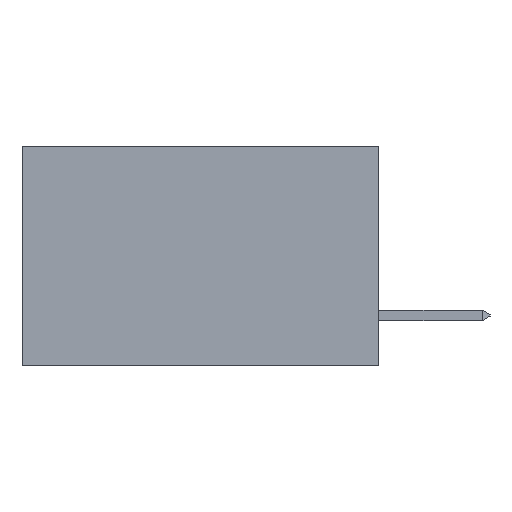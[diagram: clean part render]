
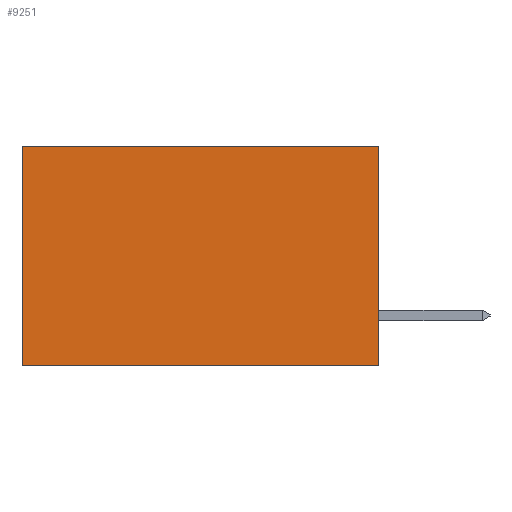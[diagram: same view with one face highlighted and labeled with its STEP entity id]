
A CAD part, left-side view. The second image highlights one B-rep face of the part: STEP entity #9251.
In plain terms, the highlighted planar face has unit normal (-1, 0, 0).
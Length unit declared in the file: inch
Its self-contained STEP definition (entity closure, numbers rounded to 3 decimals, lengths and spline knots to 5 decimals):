
#196 = VERTEX_POINT ( 'NONE', #3604 ) ;
#476 = EDGE_CURVE ( 'NONE', #13843, #8847, #13834, .T. ) ;
#494 = EDGE_CURVE ( 'NONE', #1708, #8847, #13477, .T. ) ;
#782 = VECTOR ( 'NONE', #2326, 39.37008 ) ;
#1019 = VECTOR ( 'NONE', #5736, 39.37008 ) ;
#1708 = VERTEX_POINT ( 'NONE', #10414 ) ;
#2326 = DIRECTION ( 'NONE',  ( 0., 0., -1. ) ) ;
#2496 = DIRECTION ( 'NONE',  ( 0., 1., 0. ) ) ;
#3188 = CARTESIAN_POINT ( 'NONE',  ( 0.2615, 0.6, -0.37 ) ) ;
#3313 = EDGE_CURVE ( 'NONE', #196, #13843, #5553, .T. ) ;
#3604 = CARTESIAN_POINT ( 'NONE',  ( 0.2615, 0., 0. ) ) ;
#3750 = ORIENTED_EDGE ( 'NONE', *, *, #494, .T. ) ;
#4293 = FACE_OUTER_BOUND ( 'NONE', #13920, .T. ) ;
#4460 = VECTOR ( 'NONE', #2496, 39.37008 ) ;
#4740 = DIRECTION ( 'NONE',  ( 1., 0., 0. ) ) ;
#5553 = LINE ( 'NONE', #10994, #14552 ) ;
#5736 = DIRECTION ( 'NONE',  ( 0., 1., 0. ) ) ;
#5875 = CARTESIAN_POINT ( 'NONE',  ( 0.2615, 0., -0.37 ) ) ;
#6278 = CARTESIAN_POINT ( 'NONE',  ( 0.2615, 0., -0.37 ) ) ;
#7229 = AXIS2_PLACEMENT_3D ( 'NONE', #5875, #4740, #12962 ) ;
#7521 = LINE ( 'NONE', #13962, #1019 ) ;
#8629 = EDGE_CURVE ( 'NONE', #196, #1708, #7521, .T. ) ;
#8847 = VERTEX_POINT ( 'NONE', #14300 ) ;
#9251 = ADVANCED_FACE ( 'NONE', ( #4293 ), #11771, .F. ) ;
#10414 = CARTESIAN_POINT ( 'NONE',  ( 0.2615, 0.6, 0. ) ) ;
#10704 = ORIENTED_EDGE ( 'NONE', *, *, #476, .F. ) ;
#10994 = CARTESIAN_POINT ( 'NONE',  ( 0.2615, 0., -0.37 ) ) ;
#11108 = DIRECTION ( 'NONE',  ( 0., 0., -1. ) ) ;
#11771 = PLANE ( 'NONE',  #7229 ) ;
#12962 = DIRECTION ( 'NONE',  ( 0., 0., -1. ) ) ;
#13477 = LINE ( 'NONE', #3188, #782 ) ;
#13713 = ORIENTED_EDGE ( 'NONE', *, *, #3313, .F. ) ;
#13834 = LINE ( 'NONE', #6278, #4460 ) ;
#13843 = VERTEX_POINT ( 'NONE', #14957 ) ;
#13920 = EDGE_LOOP ( 'NONE', ( #3750, #10704, #13713, #14050 ) ) ;
#13962 = CARTESIAN_POINT ( 'NONE',  ( 0.2615, 0., 0. ) ) ;
#14050 = ORIENTED_EDGE ( 'NONE', *, *, #8629, .T. ) ;
#14300 = CARTESIAN_POINT ( 'NONE',  ( 0.2615, 0.6, -0.37 ) ) ;
#14552 = VECTOR ( 'NONE', #11108, 39.37008 ) ;
#14957 = CARTESIAN_POINT ( 'NONE',  ( 0.2615, 0., -0.37 ) ) ;
